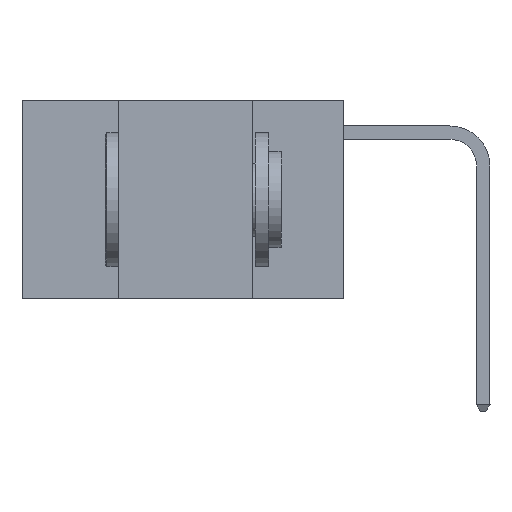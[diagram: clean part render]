
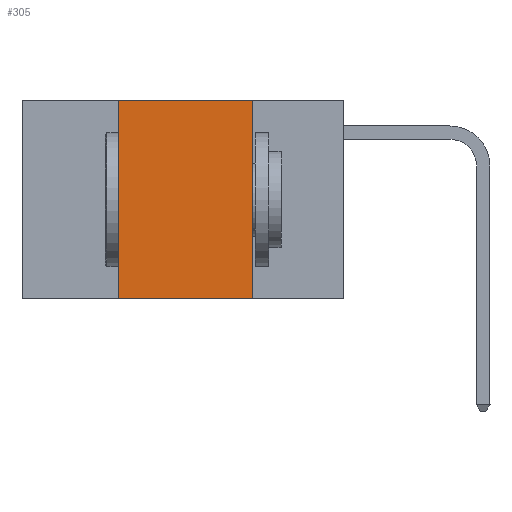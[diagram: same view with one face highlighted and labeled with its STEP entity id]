
A CAD part, left-side view. The second image highlights one B-rep face of the part: STEP entity #305.
In plain terms, the highlighted planar face has unit normal (-1, 0, 0).
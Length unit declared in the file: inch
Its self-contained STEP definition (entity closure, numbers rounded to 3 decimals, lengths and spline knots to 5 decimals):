
#305 = ADVANCED_FACE ( 'NONE', ( #4086 ), #20600, .F. ) ;
#1888 = ORIENTED_EDGE ( 'NONE', *, *, #19246, .F. ) ;
#2765 = CARTESIAN_POINT ( 'NONE',  ( 0., 0.6, 0. ) ) ;
#3245 = ORIENTED_EDGE ( 'NONE', *, *, #18263, .F. ) ;
#3348 = CARTESIAN_POINT ( 'NONE',  ( 0., 0.17, 0. ) ) ;
#3646 = VECTOR ( 'NONE', #13797, 39.37008 ) ;
#4086 = FACE_OUTER_BOUND ( 'NONE', #21575, .T. ) ;
#4510 = ORIENTED_EDGE ( 'NONE', *, *, #16948, .F. ) ;
#4677 = CARTESIAN_POINT ( 'NONE',  ( 0., 0.6, -0.37 ) ) ;
#5236 = CARTESIAN_POINT ( 'NONE',  ( 0., 0.42, 0. ) ) ;
#5678 = VERTEX_POINT ( 'NONE', #7568 ) ;
#6457 = LINE ( 'NONE', #8057, #22340 ) ;
#7568 = CARTESIAN_POINT ( 'NONE',  ( 0., 0.42, 0. ) ) ;
#7604 = EDGE_CURVE ( 'NONE', #17003, #22289, #8725, .T. ) ;
#8057 = CARTESIAN_POINT ( 'NONE',  ( 0., 0.17, 0. ) ) ;
#8725 = LINE ( 'NONE', #4677, #19282 ) ;
#8889 = ORIENTED_EDGE ( 'NONE', *, *, #7604, .T. ) ;
#9482 = CARTESIAN_POINT ( 'NONE',  ( 0., 0.42, -0.37 ) ) ;
#9667 = LINE ( 'NONE', #9776, #3646 ) ;
#9776 = CARTESIAN_POINT ( 'NONE',  ( 0., 0.6, 0. ) ) ;
#10136 = DIRECTION ( 'NONE',  ( 1., 0., 0. ) ) ;
#11170 = AXIS2_PLACEMENT_3D ( 'NONE', #2765, #10136, #12013 ) ;
#11420 = CARTESIAN_POINT ( 'NONE',  ( 0., 0.17, -0.37 ) ) ;
#12013 = DIRECTION ( 'NONE',  ( 0., 0., -1. ) ) ;
#12267 = LINE ( 'NONE', #5236, #16296 ) ;
#13797 = DIRECTION ( 'NONE',  ( 0., -1., 0. ) ) ;
#16296 = VECTOR ( 'NONE', #21175, 39.37008 ) ;
#16948 = EDGE_CURVE ( 'NONE', #17003, #5678, #12267, .T. ) ;
#17003 = VERTEX_POINT ( 'NONE', #9482 ) ;
#18263 = EDGE_CURVE ( 'NONE', #5678, #20932, #9667, .T. ) ;
#18653 = DIRECTION ( 'NONE',  ( 0., -1., 0. ) ) ;
#19246 = EDGE_CURVE ( 'NONE', #20932, #22289, #6457, .T. ) ;
#19282 = VECTOR ( 'NONE', #18653, 39.37008 ) ;
#20600 = PLANE ( 'NONE',  #11170 ) ;
#20932 = VERTEX_POINT ( 'NONE', #3348 ) ;
#21175 = DIRECTION ( 'NONE',  ( 0., 0., 1. ) ) ;
#21575 = EDGE_LOOP ( 'NONE', ( #1888, #3245, #4510, #8889 ) ) ;
#22289 = VERTEX_POINT ( 'NONE', #11420 ) ;
#22340 = VECTOR ( 'NONE', #23959, 39.37008 ) ;
#23959 = DIRECTION ( 'NONE',  ( 0., 0., -1. ) ) ;
